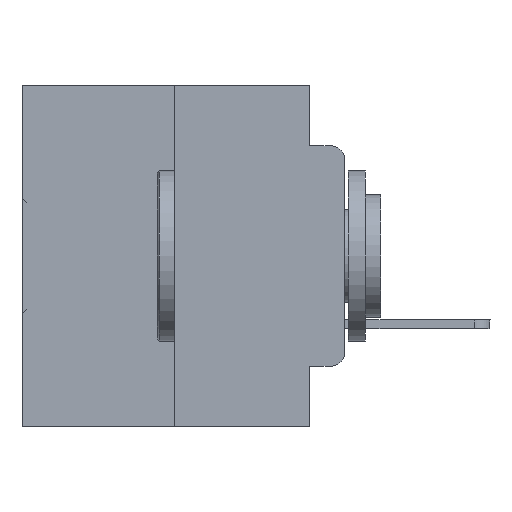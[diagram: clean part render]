
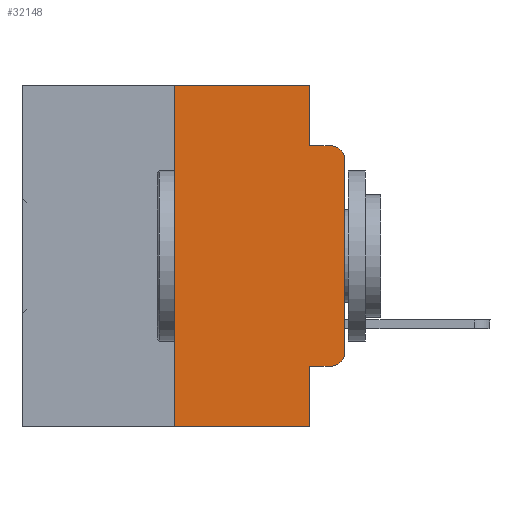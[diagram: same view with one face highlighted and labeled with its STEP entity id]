
A CAD part, left-side view. The second image highlights one B-rep face of the part: STEP entity #32148.
In plain terms, the highlighted planar face has unit normal (-1, 0, 0).
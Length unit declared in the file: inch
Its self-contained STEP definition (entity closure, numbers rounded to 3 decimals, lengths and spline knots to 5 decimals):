
#194 = EDGE_LOOP ( 'NONE', ( #1329, #33341, #2237, #15676, #11125, #12153, #9463, #4365, #27830, #32178 ) ) ;
#326 = CARTESIAN_POINT ( 'NONE',  ( 0., 0.051, -0.0885 ) ) ;
#598 = VECTOR ( 'NONE', #6687, 39.37008 ) ;
#691 = FACE_OUTER_BOUND ( 'NONE', #194, .T. ) ;
#800 = LINE ( 'NONE', #6473, #5660 ) ;
#1215 = LINE ( 'NONE', #6721, #26659 ) ;
#1242 = CARTESIAN_POINT ( 'NONE',  ( 0., 0.051, 0. ) ) ;
#1329 = ORIENTED_EDGE ( 'NONE', *, *, #33233, .T. ) ;
#1526 = CARTESIAN_POINT ( 'NONE',  ( 0., 0.473, 0. ) ) ;
#2237 = ORIENTED_EDGE ( 'NONE', *, *, #8892, .F. ) ;
#2484 = AXIS2_PLACEMENT_3D ( 'NONE', #33422, #7026, #28761 ) ;
#3215 = DIRECTION ( 'NONE',  ( 0., 0., 1. ) ) ;
#4365 = ORIENTED_EDGE ( 'NONE', *, *, #22906, .F. ) ;
#4818 = VERTEX_POINT ( 'NONE', #10286 ) ;
#5660 = VECTOR ( 'NONE', #3215, 39.37008 ) ;
#6473 = CARTESIAN_POINT ( 'NONE',  ( 0., 0., 0. ) ) ;
#6520 = LINE ( 'NONE', #1526, #598 ) ;
#6687 = DIRECTION ( 'NONE',  ( 0., -1., 0. ) ) ;
#6721 = CARTESIAN_POINT ( 'NONE',  ( 0., 0.051, -0.0885 ) ) ;
#7026 = DIRECTION ( 'NONE',  ( -1., 0., 0. ) ) ;
#7050 = CARTESIAN_POINT ( 'NONE',  ( 0., 0., -0.3915 ) ) ;
#7115 = CARTESIAN_POINT ( 'NONE',  ( 0., 0.02, -0.4115 ) ) ;
#8303 = DIRECTION ( 'NONE',  ( 0., 0., -1. ) ) ;
#8767 = DIRECTION ( 'NONE',  ( 0., 0., -1. ) ) ;
#8769 = EDGE_CURVE ( 'NONE', #17342, #18956, #20019, .T. ) ;
#8892 = EDGE_CURVE ( 'NONE', #27201, #18956, #1215, .T. ) ;
#9431 = EDGE_CURVE ( 'NONE', #33981, #24247, #30531, .T. ) ;
#9463 = ORIENTED_EDGE ( 'NONE', *, *, #11865, .T. ) ;
#10286 = CARTESIAN_POINT ( 'NONE',  ( 0., 0.051, -0.5 ) ) ;
#10391 = CARTESIAN_POINT ( 'NONE',  ( 0., 0., -0.1085 ) ) ;
#10898 = DIRECTION ( 'NONE',  ( -1., 0., 0. ) ) ;
#11125 = ORIENTED_EDGE ( 'NONE', *, *, #31055, .F. ) ;
#11732 = VERTEX_POINT ( 'NONE', #1242 ) ;
#11856 = VECTOR ( 'NONE', #14680, 39.37008 ) ;
#11865 = EDGE_CURVE ( 'NONE', #25781, #4818, #22967, .T. ) ;
#12153 = ORIENTED_EDGE ( 'NONE', *, *, #29569, .F. ) ;
#14125 = PLANE ( 'NONE',  #18918 ) ;
#14447 = VECTOR ( 'NONE', #28251, 39.37008 ) ;
#14503 = CARTESIAN_POINT ( 'NONE',  ( 0., 0.473, -0.5 ) ) ;
#14680 = DIRECTION ( 'NONE',  ( 0., -1., 0. ) ) ;
#15676 = ORIENTED_EDGE ( 'NONE', *, *, #32797, .F. ) ;
#15986 = DIRECTION ( 'NONE',  ( 0., 0., 1. ) ) ;
#16724 = VERTEX_POINT ( 'NONE', #31249 ) ;
#17342 = VERTEX_POINT ( 'NONE', #10391 ) ;
#17404 = CARTESIAN_POINT ( 'NONE',  ( 0., 0.25, -0.5 ) ) ;
#17735 = CARTESIAN_POINT ( 'NONE',  ( 0., 0.051, 0. ) ) ;
#17955 = DIRECTION ( 'NONE',  ( 0., -1., 0. ) ) ;
#18387 = AXIS2_PLACEMENT_3D ( 'NONE', #29187, #10898, #8303 ) ;
#18918 = AXIS2_PLACEMENT_3D ( 'NONE', #26745, #26919, #32261 ) ;
#18956 = VERTEX_POINT ( 'NONE', #20014 ) ;
#19420 = VECTOR ( 'NONE', #17955, 39.37008 ) ;
#19506 = DIRECTION ( 'NONE',  ( 0., -1., 0. ) ) ;
#20014 = CARTESIAN_POINT ( 'NONE',  ( 0., 0.02, -0.0885 ) ) ;
#20019 = CIRCLE ( 'NONE', #18387, 0.02 ) ;
#20429 = VECTOR ( 'NONE', #15986, 39.37008 ) ;
#21266 = VERTEX_POINT ( 'NONE', #25374 ) ;
#22226 = LINE ( 'NONE', #17735, #14447 ) ;
#22650 = EDGE_CURVE ( 'NONE', #21266, #33981, #26570, .T. ) ;
#22906 = EDGE_CURVE ( 'NONE', #21266, #4818, #22226, .T. ) ;
#22967 = LINE ( 'NONE', #14503, #11856 ) ;
#24247 = VERTEX_POINT ( 'NONE', #7050 ) ;
#24367 = VECTOR ( 'NONE', #8767, 39.37008 ) ;
#24805 = LINE ( 'NONE', #27065, #24367 ) ;
#25374 = CARTESIAN_POINT ( 'NONE',  ( 0., 0.051, -0.4115 ) ) ;
#25781 = VERTEX_POINT ( 'NONE', #17404 ) ;
#26570 = LINE ( 'NONE', #29161, #19420 ) ;
#26659 = VECTOR ( 'NONE', #19506, 39.37008 ) ;
#26745 = CARTESIAN_POINT ( 'NONE',  ( 0., 0.473, 0. ) ) ;
#26919 = DIRECTION ( 'NONE',  ( 1., 0., 0. ) ) ;
#27065 = CARTESIAN_POINT ( 'NONE',  ( 0., 0.051, 0. ) ) ;
#27201 = VERTEX_POINT ( 'NONE', #326 ) ;
#27830 = ORIENTED_EDGE ( 'NONE', *, *, #22650, .T. ) ;
#28251 = DIRECTION ( 'NONE',  ( 0., 0., -1. ) ) ;
#28761 = DIRECTION ( 'NONE',  ( 0., 0., -1. ) ) ;
#29103 = CARTESIAN_POINT ( 'NONE',  ( 0., 0.25, 0. ) ) ;
#29161 = CARTESIAN_POINT ( 'NONE',  ( 0., 0.051, -0.4115 ) ) ;
#29187 = CARTESIAN_POINT ( 'NONE',  ( 0., 0.02, -0.1085 ) ) ;
#29569 = EDGE_CURVE ( 'NONE', #25781, #16724, #32200, .T. ) ;
#30531 = CIRCLE ( 'NONE', #2484, 0.02 ) ;
#31055 = EDGE_CURVE ( 'NONE', #16724, #11732, #6520, .T. ) ;
#31249 = CARTESIAN_POINT ( 'NONE',  ( 0., 0.25, 0. ) ) ;
#32148 = ADVANCED_FACE ( 'NONE', ( #691 ), #14125, .F. ) ;
#32178 = ORIENTED_EDGE ( 'NONE', *, *, #9431, .T. ) ;
#32200 = LINE ( 'NONE', #29103, #20429 ) ;
#32261 = DIRECTION ( 'NONE',  ( 0., 0., -1. ) ) ;
#32797 = EDGE_CURVE ( 'NONE', #11732, #27201, #24805, .T. ) ;
#33233 = EDGE_CURVE ( 'NONE', #24247, #17342, #800, .T. ) ;
#33341 = ORIENTED_EDGE ( 'NONE', *, *, #8769, .T. ) ;
#33422 = CARTESIAN_POINT ( 'NONE',  ( 0., 0.02, -0.3915 ) ) ;
#33981 = VERTEX_POINT ( 'NONE', #7115 ) ;
